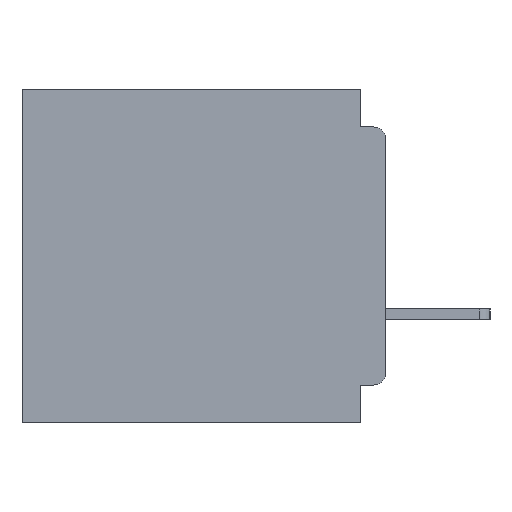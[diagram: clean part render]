
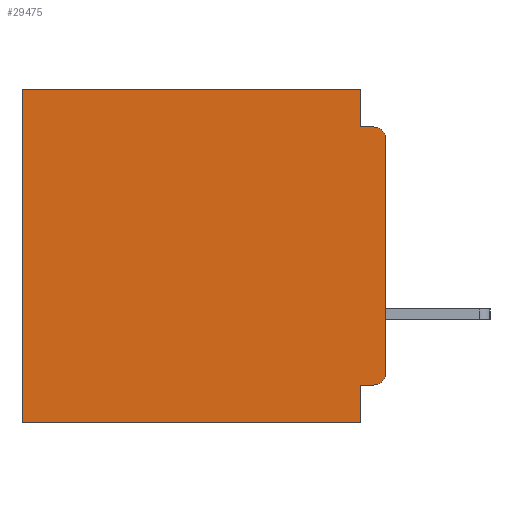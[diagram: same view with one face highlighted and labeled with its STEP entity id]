
A CAD part, left-side view. The second image highlights one B-rep face of the part: STEP entity #29475.
In plain terms, the highlighted planar face has unit normal (-1, 0, 0).
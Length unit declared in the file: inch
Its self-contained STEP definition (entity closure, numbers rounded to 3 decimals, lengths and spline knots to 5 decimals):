
#455 = EDGE_LOOP ( 'NONE', ( #12032, #21580, #31983, #33647, #22014, #19084, #6626, #8305, #1996, #27445 ) ) ;
#537 = CARTESIAN_POINT ( 'NONE',  ( 0.3, 0., -0.4 ) ) ;
#960 = VECTOR ( 'NONE', #30331, 39.37008 ) ;
#1027 = VERTEX_POINT ( 'NONE', #22605 ) ;
#1996 = ORIENTED_EDGE ( 'NONE', *, *, #16406, .F. ) ;
#2254 = DIRECTION ( 'NONE',  ( 0., 0., -1. ) ) ;
#2342 = DIRECTION ( 'NONE',  ( -1., 0., 0. ) ) ;
#3471 = CARTESIAN_POINT ( 'NONE',  ( 0.3, 0.031, -0.4 ) ) ;
#3754 = VECTOR ( 'NONE', #19762, 39.37008 ) ;
#4034 = DIRECTION ( 'NONE',  ( 1., 0., 0. ) ) ;
#4065 = VERTEX_POINT ( 'NONE', #18790 ) ;
#4166 = AXIS2_PLACEMENT_3D ( 'NONE', #18314, #2342, #21006 ) ;
#4628 = EDGE_CURVE ( 'NONE', #31560, #14039, #13197, .T. ) ;
#6013 = CARTESIAN_POINT ( 'NONE',  ( 0.3, 0., -0.045 ) ) ;
#6199 = DIRECTION ( 'NONE',  ( 0., 0., -1. ) ) ;
#6310 = VERTEX_POINT ( 'NONE', #19681 ) ;
#6626 = ORIENTED_EDGE ( 'NONE', *, *, #32469, .F. ) ;
#7490 = CARTESIAN_POINT ( 'NONE',  ( 0.3, 0.437, 0. ) ) ;
#7757 = CIRCLE ( 'NONE', #4166, 0.015 ) ;
#8305 = ORIENTED_EDGE ( 'NONE', *, *, #23988, .F. ) ;
#9071 = CARTESIAN_POINT ( 'NONE',  ( 0.3, 0., -0.4 ) ) ;
#9317 = CARTESIAN_POINT ( 'NONE',  ( 0.3, 0., -0.4 ) ) ;
#10083 = VERTEX_POINT ( 'NONE', #28816 ) ;
#10513 = LINE ( 'NONE', #10663, #30880 ) ;
#10663 = CARTESIAN_POINT ( 'NONE',  ( 0.3, 0., -0.355 ) ) ;
#11053 = VECTOR ( 'NONE', #29977, 39.37008 ) ;
#11337 = CARTESIAN_POINT ( 'NONE',  ( 0.3, 0., -0.06 ) ) ;
#12032 = ORIENTED_EDGE ( 'NONE', *, *, #27282, .F. ) ;
#12453 = CARTESIAN_POINT ( 'NONE',  ( 0.3, 0.437, -0.4 ) ) ;
#12459 = LINE ( 'NONE', #537, #32819 ) ;
#12497 = EDGE_CURVE ( 'NONE', #15422, #31560, #23096, .T. ) ;
#13197 = LINE ( 'NONE', #12453, #24819 ) ;
#13376 = DIRECTION ( 'NONE',  ( 0., 1., 0. ) ) ;
#14039 = VERTEX_POINT ( 'NONE', #20490 ) ;
#15422 = VERTEX_POINT ( 'NONE', #34558 ) ;
#15574 = VERTEX_POINT ( 'NONE', #11337 ) ;
#16406 = EDGE_CURVE ( 'NONE', #27443, #28028, #10513, .T. ) ;
#16687 = DIRECTION ( 'NONE',  ( 0., 0., -1. ) ) ;
#17875 = LINE ( 'NONE', #30676, #31181 ) ;
#17879 = AXIS2_PLACEMENT_3D ( 'NONE', #34146, #18233, #2254 ) ;
#17944 = EDGE_CURVE ( 'NONE', #15422, #10083, #17875, .T. ) ;
#18104 = LINE ( 'NONE', #6013, #11053 ) ;
#18233 = DIRECTION ( 'NONE',  ( -1., 0., 0. ) ) ;
#18314 = CARTESIAN_POINT ( 'NONE',  ( 0.3, 0.015, -0.34 ) ) ;
#18790 = CARTESIAN_POINT ( 'NONE',  ( 0.3, 0.015, -0.045 ) ) ;
#19041 = LINE ( 'NONE', #3471, #32377 ) ;
#19084 = ORIENTED_EDGE ( 'NONE', *, *, #4628, .T. ) ;
#19681 = CARTESIAN_POINT ( 'NONE',  ( 0.3, 0.031, -0.4 ) ) ;
#19762 = DIRECTION ( 'NONE',  ( 0., 1., 0. ) ) ;
#20103 = EDGE_CURVE ( 'NONE', #15574, #4065, #21399, .T. ) ;
#20167 = CARTESIAN_POINT ( 'NONE',  ( 0.3, 0.015, -0.355 ) ) ;
#20490 = CARTESIAN_POINT ( 'NONE',  ( 0.3, 0.437, -0.4 ) ) ;
#21006 = DIRECTION ( 'NONE',  ( 0., 0., -1. ) ) ;
#21399 = CIRCLE ( 'NONE', #17879, 0.015 ) ;
#21580 = ORIENTED_EDGE ( 'NONE', *, *, #20103, .T. ) ;
#22014 = ORIENTED_EDGE ( 'NONE', *, *, #12497, .T. ) ;
#22605 = CARTESIAN_POINT ( 'NONE',  ( 0.3, 0., -0.34 ) ) ;
#22691 = DIRECTION ( 'NONE',  ( 0., 0., -1. ) ) ;
#23096 = LINE ( 'NONE', #24998, #960 ) ;
#23636 = AXIS2_PLACEMENT_3D ( 'NONE', #9317, #4034, #22691 ) ;
#23988 = EDGE_CURVE ( 'NONE', #28028, #6310, #19041, .T. ) ;
#24819 = VECTOR ( 'NONE', #27950, 39.37008 ) ;
#24998 = CARTESIAN_POINT ( 'NONE',  ( 0.3, 0., 0. ) ) ;
#25053 = LINE ( 'NONE', #9071, #3754 ) ;
#27282 = EDGE_CURVE ( 'NONE', #15574, #1027, #12459, .T. ) ;
#27443 = VERTEX_POINT ( 'NONE', #20167 ) ;
#27445 = ORIENTED_EDGE ( 'NONE', *, *, #28557, .T. ) ;
#27935 = PLANE ( 'NONE',  #23636 ) ;
#27950 = DIRECTION ( 'NONE',  ( 0., 0., -1. ) ) ;
#28028 = VERTEX_POINT ( 'NONE', #29410 ) ;
#28557 = EDGE_CURVE ( 'NONE', #27443, #1027, #7757, .T. ) ;
#28816 = CARTESIAN_POINT ( 'NONE',  ( 0.3, 0.031, -0.045 ) ) ;
#29410 = CARTESIAN_POINT ( 'NONE',  ( 0.3, 0.031, -0.355 ) ) ;
#29475 = ADVANCED_FACE ( 'NONE', ( #33946 ), #27935, .F. ) ;
#29923 = EDGE_CURVE ( 'NONE', #10083, #4065, #18104, .T. ) ;
#29977 = DIRECTION ( 'NONE',  ( 0., -1., 0. ) ) ;
#30331 = DIRECTION ( 'NONE',  ( 0., 1., 0. ) ) ;
#30676 = CARTESIAN_POINT ( 'NONE',  ( 0.3, 0.031, 0. ) ) ;
#30880 = VECTOR ( 'NONE', #13376, 39.37008 ) ;
#31181 = VECTOR ( 'NONE', #33333, 39.37008 ) ;
#31560 = VERTEX_POINT ( 'NONE', #7490 ) ;
#31983 = ORIENTED_EDGE ( 'NONE', *, *, #29923, .F. ) ;
#32377 = VECTOR ( 'NONE', #6199, 39.37008 ) ;
#32469 = EDGE_CURVE ( 'NONE', #6310, #14039, #25053, .T. ) ;
#32819 = VECTOR ( 'NONE', #16687, 39.37008 ) ;
#33333 = DIRECTION ( 'NONE',  ( 0., 0., -1. ) ) ;
#33647 = ORIENTED_EDGE ( 'NONE', *, *, #17944, .F. ) ;
#33946 = FACE_OUTER_BOUND ( 'NONE', #455, .T. ) ;
#34146 = CARTESIAN_POINT ( 'NONE',  ( 0.3, 0.015, -0.06 ) ) ;
#34558 = CARTESIAN_POINT ( 'NONE',  ( 0.3, 0.031, 0. ) ) ;
